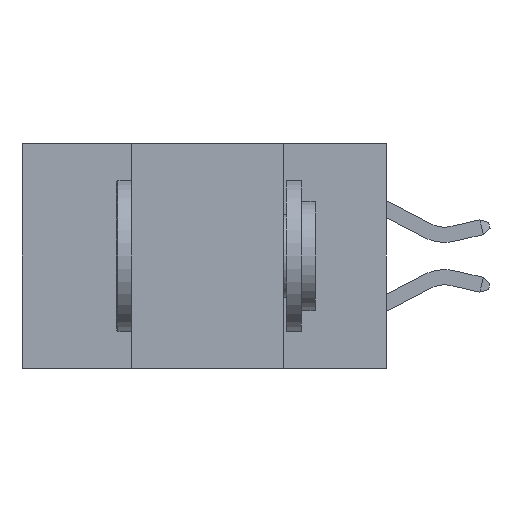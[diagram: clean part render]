
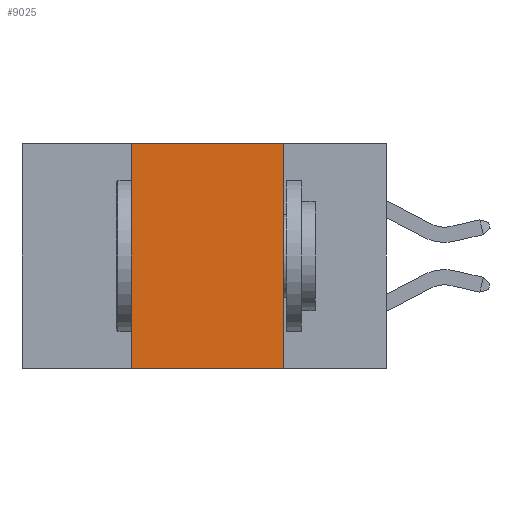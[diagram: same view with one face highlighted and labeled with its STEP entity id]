
A CAD part, left-side view. The second image highlights one B-rep face of the part: STEP entity #9025.
In plain terms, the highlighted planar face has unit normal (-1, 0, 0).
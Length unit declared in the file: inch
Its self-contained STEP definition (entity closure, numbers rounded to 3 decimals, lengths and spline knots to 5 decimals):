
#899 = VECTOR ( 'NONE', #17786, 39.37008 ) ;
#3465 = VERTEX_POINT ( 'NONE', #17595 ) ;
#5659 = DIRECTION ( 'NONE',  ( 0., 0., -1. ) ) ;
#5971 = ORIENTED_EDGE ( 'NONE', *, *, #6622, .F. ) ;
#6083 = CARTESIAN_POINT ( 'NONE',  ( 0., 0.42, 0. ) ) ;
#6283 = LINE ( 'NONE', #21314, #6492 ) ;
#6492 = VECTOR ( 'NONE', #14064, 39.37008 ) ;
#6622 = EDGE_CURVE ( 'NONE', #11385, #3465, #20204, .T. ) ;
#7141 = VECTOR ( 'NONE', #5659, 39.37008 ) ;
#8971 = CARTESIAN_POINT ( 'NONE',  ( 0., 0.6, 0. ) ) ;
#9025 = ADVANCED_FACE ( 'NONE', ( #12643 ), #12524, .F. ) ;
#11005 = EDGE_CURVE ( 'NONE', #23671, #11385, #6283, .T. ) ;
#11385 = VERTEX_POINT ( 'NONE', #15163 ) ;
#11498 = EDGE_CURVE ( 'NONE', #15276, #23671, #12687, .T. ) ;
#11774 = LINE ( 'NONE', #21561, #11844 ) ;
#11844 = VECTOR ( 'NONE', #19503, 39.37008 ) ;
#12524 = PLANE ( 'NONE',  #18936 ) ;
#12643 = FACE_OUTER_BOUND ( 'NONE', #15924, .T. ) ;
#12677 = ORIENTED_EDGE ( 'NONE', *, *, #14115, .T. ) ;
#12687 = LINE ( 'NONE', #21894, #899 ) ;
#14064 = DIRECTION ( 'NONE',  ( 0., -1., 0. ) ) ;
#14115 = EDGE_CURVE ( 'NONE', #15276, #3465, #11774, .T. ) ;
#14365 = DIRECTION ( 'NONE',  ( 1., 0., 0. ) ) ;
#15163 = CARTESIAN_POINT ( 'NONE',  ( 0., 0.17, 0. ) ) ;
#15276 = VERTEX_POINT ( 'NONE', #20497 ) ;
#15924 = EDGE_LOOP ( 'NONE', ( #5971, #19228, #18999, #12677 ) ) ;
#17595 = CARTESIAN_POINT ( 'NONE',  ( 0., 0.17, -0.37 ) ) ;
#17786 = DIRECTION ( 'NONE',  ( 0., 0., 1. ) ) ;
#18936 = AXIS2_PLACEMENT_3D ( 'NONE', #8971, #14365, #20015 ) ;
#18999 = ORIENTED_EDGE ( 'NONE', *, *, #11498, .F. ) ;
#19228 = ORIENTED_EDGE ( 'NONE', *, *, #11005, .F. ) ;
#19503 = DIRECTION ( 'NONE',  ( 0., -1., 0. ) ) ;
#20015 = DIRECTION ( 'NONE',  ( 0., 0., -1. ) ) ;
#20204 = LINE ( 'NONE', #20575, #7141 ) ;
#20497 = CARTESIAN_POINT ( 'NONE',  ( 0., 0.42, -0.37 ) ) ;
#20575 = CARTESIAN_POINT ( 'NONE',  ( 0., 0.17, -0.37 ) ) ;
#21314 = CARTESIAN_POINT ( 'NONE',  ( 0., 0.6, 0. ) ) ;
#21561 = CARTESIAN_POINT ( 'NONE',  ( 0., 0.6, -0.37 ) ) ;
#21894 = CARTESIAN_POINT ( 'NONE',  ( 0., 0.42, -0.37 ) ) ;
#23671 = VERTEX_POINT ( 'NONE', #6083 ) ;
